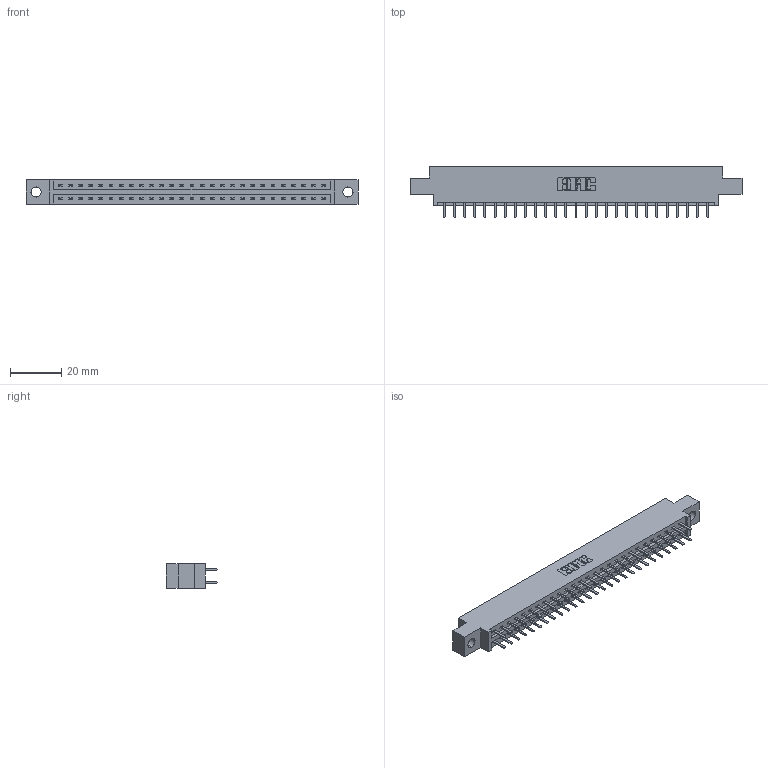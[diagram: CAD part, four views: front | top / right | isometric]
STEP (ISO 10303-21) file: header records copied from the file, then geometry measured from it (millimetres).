
FILE_DESCRIPTION (( 'STEP AP203' ), '1' );
FILE_NAME ('337-054-520-804.STEP', '2018-08-10T00:10:14', ( '' ), ( '' ), 'SwSTEP 2.0', 'SolidWorks 2016', '' );
FILE_SCHEMA (( 'CONFIG_CONTROL_DESIGN' ));
Length unit declared in the file: inch
Products named in the file (3): 345-292-001_345-293-120; 337-054-520-804; 337 Part_0.170 Offset - 0.156 Dia-TH
Assembly tree (55 placements, depth 2):
  337-054-520-804
    337 Part_0.170 Offset - 0.156 Dia-TH
    345-292-001_345-293-120  x54
Bounding box: 130 x 20.02 x 9.4 mm (x, y, z)
Volume: 13271.4 mm3; surface area: 14695.1 mm2
Topology: 55 solids, 55 shells, 3250 faces, 9449 edges, 6154 vertices
Faces by surface type: plane 2234, cylinder 1016
Entity records: 23123 total; most frequent: CARTESIAN_POINT 3922, ORIENTED_EDGE 3846, DIRECTION 3351, EDGE_CURVE 1923, LINE 1791, VECTOR 1791, VERTEX_POINT 1278, AXIS2_PLACEMENT_3D 780
